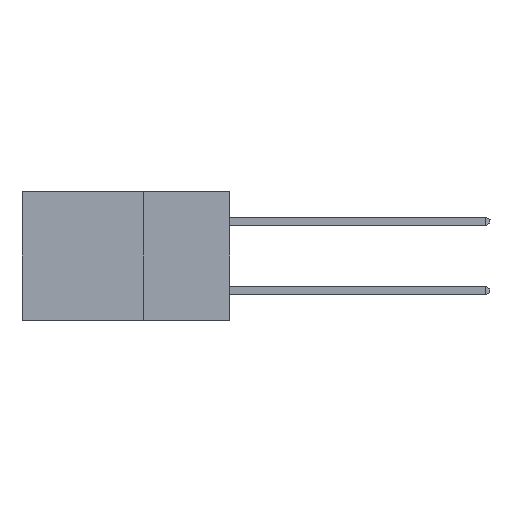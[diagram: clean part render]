
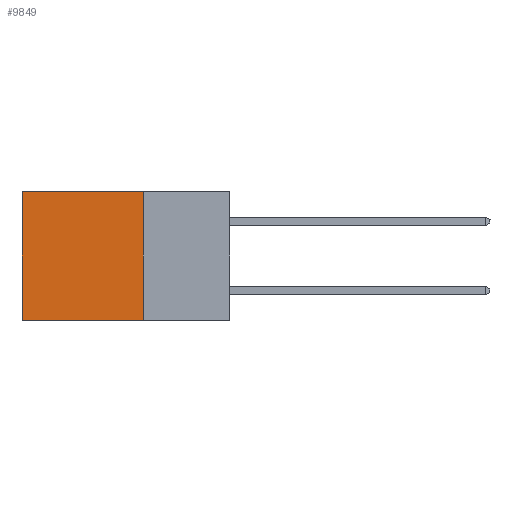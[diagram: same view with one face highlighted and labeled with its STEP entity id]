
A CAD part, left-side view. The second image highlights one B-rep face of the part: STEP entity #9849.
In plain terms, the highlighted planar face has unit normal (-1, 0, 0).
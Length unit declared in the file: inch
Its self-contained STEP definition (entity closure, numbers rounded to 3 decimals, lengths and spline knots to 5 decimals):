
#182 = ORIENTED_EDGE ( 'NONE', *, *, #17997, .T. ) ;
#234 = VECTOR ( 'NONE', #13314, 39.37008 ) ;
#1895 = VECTOR ( 'NONE', #10013, 39.37008 ) ;
#2062 = CARTESIAN_POINT ( 'NONE',  ( 0.298, 0.25, -0.37 ) ) ;
#2553 = AXIS2_PLACEMENT_3D ( 'NONE', #26311, #11500, #6303 ) ;
#3529 = CARTESIAN_POINT ( 'NONE',  ( 0.298, 0.25, 0. ) ) ;
#4041 = VERTEX_POINT ( 'NONE', #2062 ) ;
#4369 = EDGE_LOOP ( 'NONE', ( #182, #22787, #5810, #31716 ) ) ;
#4831 = FACE_OUTER_BOUND ( 'NONE', #4369, .T. ) ;
#5810 = ORIENTED_EDGE ( 'NONE', *, *, #29468, .F. ) ;
#6052 = DIRECTION ( 'NONE',  ( 0., 0., -1. ) ) ;
#6303 = DIRECTION ( 'NONE',  ( 0., 0., -1. ) ) ;
#6836 = LINE ( 'NONE', #30447, #234 ) ;
#7485 = VERTEX_POINT ( 'NONE', #20959 ) ;
#9849 = ADVANCED_FACE ( 'NONE', ( #4831 ), #30926, .F. ) ;
#10013 = DIRECTION ( 'NONE',  ( 0., 1., 0. ) ) ;
#11500 = DIRECTION ( 'NONE',  ( 1., 0., 0. ) ) ;
#13314 = DIRECTION ( 'NONE',  ( 0., 0., -1. ) ) ;
#14099 = LINE ( 'NONE', #16585, #29446 ) ;
#16585 = CARTESIAN_POINT ( 'NONE',  ( 0.298, 0.25, -0.37 ) ) ;
#16905 = DIRECTION ( 'NONE',  ( 0., 1., 0. ) ) ;
#17419 = CARTESIAN_POINT ( 'NONE',  ( 0.298, 0.25, 0. ) ) ;
#17997 = EDGE_CURVE ( 'NONE', #28666, #29435, #6836, .T. ) ;
#20959 = CARTESIAN_POINT ( 'NONE',  ( 0.298, 0.25, 0. ) ) ;
#22787 = ORIENTED_EDGE ( 'NONE', *, *, #25867, .F. ) ;
#24978 = LINE ( 'NONE', #3529, #25757 ) ;
#25330 = CARTESIAN_POINT ( 'NONE',  ( 0.298, 0.6, 0. ) ) ;
#25757 = VECTOR ( 'NONE', #6052, 39.37008 ) ;
#25867 = EDGE_CURVE ( 'NONE', #4041, #29435, #14099, .T. ) ;
#26311 = CARTESIAN_POINT ( 'NONE',  ( 0.298, 0.25, 0. ) ) ;
#28666 = VERTEX_POINT ( 'NONE', #25330 ) ;
#29130 = EDGE_CURVE ( 'NONE', #7485, #28666, #30749, .T. ) ;
#29435 = VERTEX_POINT ( 'NONE', #30586 ) ;
#29446 = VECTOR ( 'NONE', #16905, 39.37008 ) ;
#29468 = EDGE_CURVE ( 'NONE', #7485, #4041, #24978, .T. ) ;
#30447 = CARTESIAN_POINT ( 'NONE',  ( 0.298, 0.6, 0. ) ) ;
#30586 = CARTESIAN_POINT ( 'NONE',  ( 0.298, 0.6, -0.37 ) ) ;
#30749 = LINE ( 'NONE', #17419, #1895 ) ;
#30926 = PLANE ( 'NONE',  #2553 ) ;
#31716 = ORIENTED_EDGE ( 'NONE', *, *, #29130, .T. ) ;
